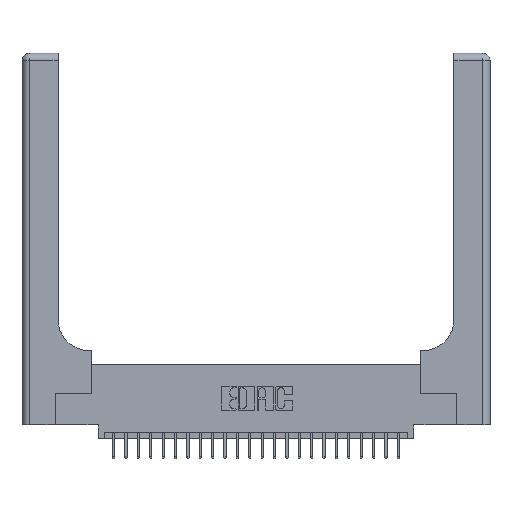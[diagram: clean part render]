
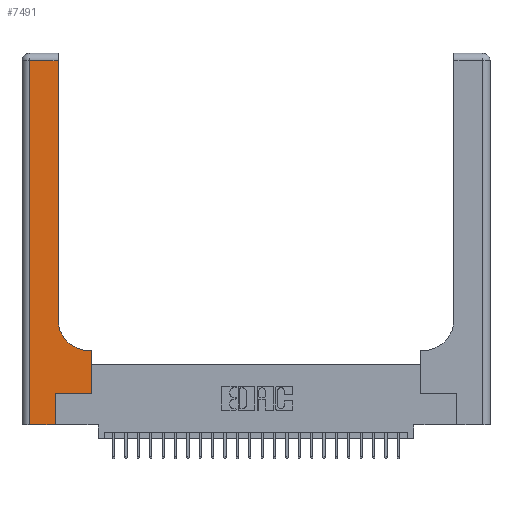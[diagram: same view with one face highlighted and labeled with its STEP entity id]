
A CAD part, top view. The second image highlights one B-rep face of the part: STEP entity #7491.
In plain terms, the highlighted planar face has unit normal (0, 0, 1).
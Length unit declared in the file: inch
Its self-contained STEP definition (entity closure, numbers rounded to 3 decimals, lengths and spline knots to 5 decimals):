
#19 = VERTEX_POINT ( 'NONE', #25883 ) ;
#1401 = LINE ( 'NONE', #19476, #16625 ) ;
#1501 = VECTOR ( 'NONE', #17255, 39.37008 ) ;
#1652 = LINE ( 'NONE', #25906, #6593 ) ;
#2510 = VERTEX_POINT ( 'NONE', #13987 ) ;
#3090 = VERTEX_POINT ( 'NONE', #12459 ) ;
#3263 = VECTOR ( 'NONE', #10782, 39.37008 ) ;
#4941 = CARTESIAN_POINT ( 'NONE',  ( 0.5415, 0.6, 0.37 ) ) ;
#4976 = CARTESIAN_POINT ( 'NONE',  ( 0.2915, 3., 0.37 ) ) ;
#5599 = DIRECTION ( 'NONE',  ( 1., 0., 0. ) ) ;
#5759 = VERTEX_POINT ( 'NONE', #13835 ) ;
#5943 = CARTESIAN_POINT ( 'NONE',  ( 0.06, 3., 0.37 ) ) ;
#6593 = VECTOR ( 'NONE', #9703, 39.37008 ) ;
#6594 = ORIENTED_EDGE ( 'NONE', *, *, #13330, .T. ) ;
#7031 = VERTEX_POINT ( 'NONE', #17953 ) ;
#7113 = DIRECTION ( 'NONE',  ( 0., 1., 0. ) ) ;
#7273 = VECTOR ( 'NONE', #12103, 39.37008 ) ;
#7491 = ADVANCED_FACE ( 'NONE', ( #25569 ), #21653, .F. ) ;
#7595 = EDGE_CURVE ( 'NONE', #23790, #19, #12852, .T. ) ;
#9452 = DIRECTION ( 'NONE',  ( 0., 0., -1. ) ) ;
#9703 = DIRECTION ( 'NONE',  ( -1., 0., 0. ) ) ;
#10043 = ORIENTED_EDGE ( 'NONE', *, *, #19352, .T. ) ;
#10206 = ORIENTED_EDGE ( 'NONE', *, *, #12833, .T. ) ;
#10398 = CARTESIAN_POINT ( 'NONE',  ( 0.5415, 0.85, 0.37 ) ) ;
#10782 = DIRECTION ( 'NONE',  ( 0., 1., 0. ) ) ;
#11190 = CARTESIAN_POINT ( 'NONE',  ( 0., 2.94, 0.37 ) ) ;
#11694 = ORIENTED_EDGE ( 'NONE', *, *, #16710, .T. ) ;
#11783 = CARTESIAN_POINT ( 'NONE',  ( 0., 0., 0.37 ) ) ;
#12103 = DIRECTION ( 'NONE',  ( 0., -1., 0. ) ) ;
#12334 = CIRCLE ( 'NONE', #19658, 0.25 ) ;
#12416 = ORIENTED_EDGE ( 'NONE', *, *, #23097, .T. ) ;
#12459 = CARTESIAN_POINT ( 'NONE',  ( 0.2915, 2.94, 0.37 ) ) ;
#12466 = DIRECTION ( 'NONE',  ( 1., 0., 0. ) ) ;
#12833 = EDGE_CURVE ( 'NONE', #19, #24096, #19051, .T. ) ;
#12852 = LINE ( 'NONE', #11783, #17623 ) ;
#13330 = EDGE_CURVE ( 'NONE', #18200, #2510, #12334, .T. ) ;
#13835 = CARTESIAN_POINT ( 'NONE',  ( 0.5585, 0.25, 0.37 ) ) ;
#13987 = CARTESIAN_POINT ( 'NONE',  ( 0.2915, 0.85, 0.37 ) ) ;
#14409 = VECTOR ( 'NONE', #19287, 39.37008 ) ;
#16625 = VECTOR ( 'NONE', #21513, 39.37008 ) ;
#16710 = EDGE_CURVE ( 'NONE', #24096, #5759, #25217, .T. ) ;
#16878 = AXIS2_PLACEMENT_3D ( 'NONE', #25649, #9452, #23726 ) ;
#17250 = CARTESIAN_POINT ( 'NONE',  ( 0.269, 0.25, 0.37 ) ) ;
#17255 = DIRECTION ( 'NONE',  ( -1., 0., 0. ) ) ;
#17372 = VECTOR ( 'NONE', #7113, 39.37008 ) ;
#17623 = VECTOR ( 'NONE', #5599, 39.37008 ) ;
#17953 = CARTESIAN_POINT ( 'NONE',  ( 0.06, 2.94, 0.37 ) ) ;
#18000 = LINE ( 'NONE', #4976, #17372 ) ;
#18200 = VERTEX_POINT ( 'NONE', #4941 ) ;
#18209 = CARTESIAN_POINT ( 'NONE',  ( 0.06, 0., 0.37 ) ) ;
#19051 = LINE ( 'NONE', #25042, #3263 ) ;
#19287 = DIRECTION ( 'NONE',  ( 1., 0., 0. ) ) ;
#19352 = EDGE_CURVE ( 'NONE', #3090, #7031, #23432, .T. ) ;
#19355 = EDGE_CURVE ( 'NONE', #2510, #3090, #18000, .T. ) ;
#19476 = CARTESIAN_POINT ( 'NONE',  ( 0.5585, 0.25, 0.37 ) ) ;
#19658 = AXIS2_PLACEMENT_3D ( 'NONE', #10398, #24651, #12466 ) ;
#20449 = CARTESIAN_POINT ( 'NONE',  ( 0.5585, 0.6, 0.37 ) ) ;
#21385 = CARTESIAN_POINT ( 'NONE',  ( 0.269, 0.25, 0.37 ) ) ;
#21513 = DIRECTION ( 'NONE',  ( 0., 1., 0. ) ) ;
#21653 = PLANE ( 'NONE',  #16878 ) ;
#21887 = EDGE_CURVE ( 'NONE', #7031, #23790, #23608, .T. ) ;
#21935 = VERTEX_POINT ( 'NONE', #20449 ) ;
#22496 = ORIENTED_EDGE ( 'NONE', *, *, #21887, .T. ) ;
#22649 = EDGE_LOOP ( 'NONE', ( #26572, #10043, #22496, #25405, #10206, #11694, #23434, #12416, #6594 ) ) ;
#23097 = EDGE_CURVE ( 'NONE', #21935, #18200, #1652, .T. ) ;
#23432 = LINE ( 'NONE', #11190, #1501 ) ;
#23434 = ORIENTED_EDGE ( 'NONE', *, *, #25202, .T. ) ;
#23608 = LINE ( 'NONE', #5943, #7273 ) ;
#23726 = DIRECTION ( 'NONE',  ( -1., 0., 0. ) ) ;
#23790 = VERTEX_POINT ( 'NONE', #18209 ) ;
#24096 = VERTEX_POINT ( 'NONE', #21385 ) ;
#24651 = DIRECTION ( 'NONE',  ( 0., 0., -1. ) ) ;
#25042 = CARTESIAN_POINT ( 'NONE',  ( 0.269, 0., 0.37 ) ) ;
#25202 = EDGE_CURVE ( 'NONE', #5759, #21935, #1401, .T. ) ;
#25217 = LINE ( 'NONE', #17250, #14409 ) ;
#25405 = ORIENTED_EDGE ( 'NONE', *, *, #7595, .T. ) ;
#25569 = FACE_OUTER_BOUND ( 'NONE', #22649, .T. ) ;
#25649 = CARTESIAN_POINT ( 'NONE',  ( 0., 3., 0.37 ) ) ;
#25883 = CARTESIAN_POINT ( 'NONE',  ( 0.269, 0., 0.37 ) ) ;
#25906 = CARTESIAN_POINT ( 'NONE',  ( 0.2915, 0.6, 0.37 ) ) ;
#26572 = ORIENTED_EDGE ( 'NONE', *, *, #19355, .T. ) ;
